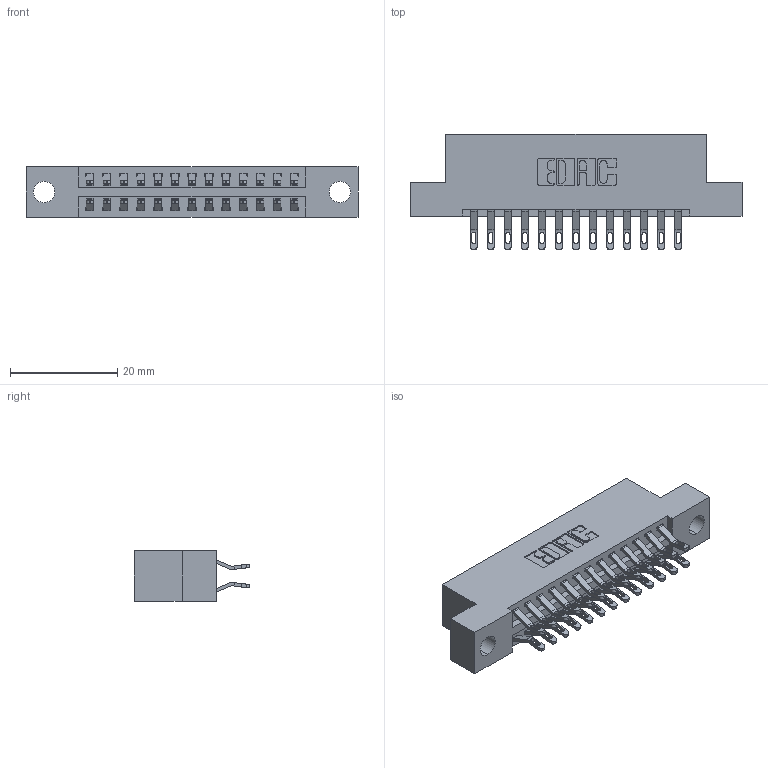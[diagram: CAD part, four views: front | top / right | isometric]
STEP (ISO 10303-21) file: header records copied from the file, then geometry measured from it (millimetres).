
FILE_DESCRIPTION (( 'STEP AP203' ), '1' );
FILE_NAME ('346-026-555-204.STEP', '2022-05-19T02:16:55', ( '' ), ( '' ), 'SwSTEP 2.0', 'SolidWorks 2020', '' );
FILE_SCHEMA (( 'CONFIG_CONTROL_DESIGN' ));
Length unit declared in the file: inch
Products named in the file (3): 345-292-001_555 Tail; 346 Part_Flush Mounting Lugs - 0.156 Dia-TH; 346-026-555-204
Assembly tree (27 placements, depth 2):
  346-026-555-204
    346 Part_Flush Mounting Lugs - 0.156 Dia-TH
    345-292-001_555 Tail  x26
Bounding box: 61.85 x 21.46 x 9.4 mm (x, y, z)
Volume: 5775.3 mm3; surface area: 7599.4 mm2
Topology: 27 solids, 27 shells, 1644 faces, 5123 edges, 3414 vertices
Faces by surface type: plane 948, cylinder 696
Entity records: 13133 total; most frequent: CARTESIAN_POINT 2244, ORIENTED_EDGE 2146, DIRECTION 1997, EDGE_CURVE 1073, LINE 869, VECTOR 869, VERTEX_POINT 714, AXIS2_PLACEMENT_3D 564
